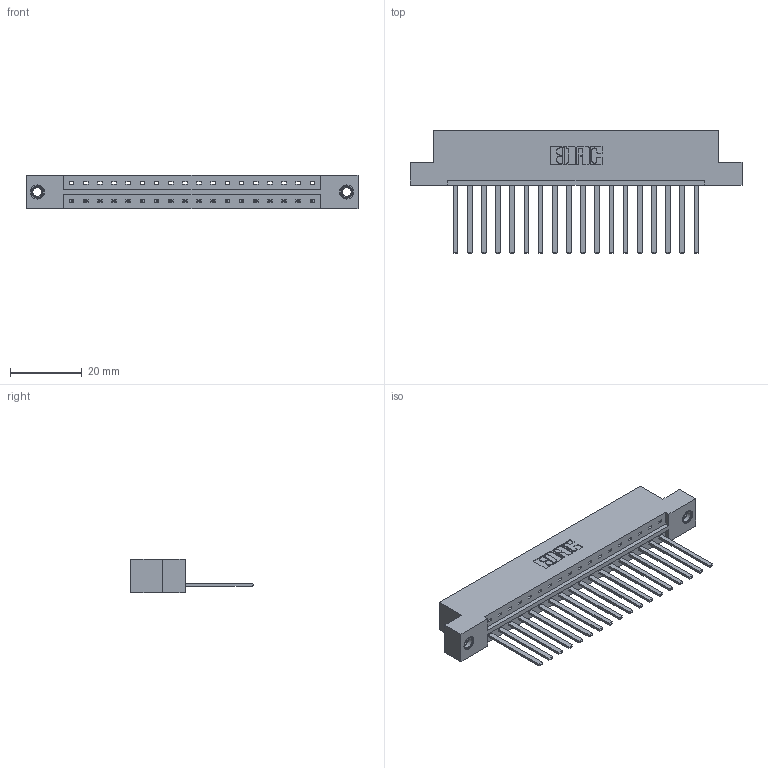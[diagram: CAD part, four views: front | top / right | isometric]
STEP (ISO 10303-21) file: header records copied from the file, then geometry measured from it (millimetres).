
FILE_DESCRIPTION (( 'STEP AP203' ), '1' );
FILE_NAME ('833-018-544-107.STEP', '2020-05-31T22:41:54', ( '' ), ( '' ), 'SwSTEP 2.0', 'SolidWorks 2020', '' );
FILE_SCHEMA (( 'CONFIG_CONTROL_DESIGN' ));
Length unit declared in the file: inch
Products named in the file (4): 833-018-544-107; 345-250-001_345-250-005-103; 833 Part_Flush - .156 Dia - TI; 345-292-001_345-293-144
Assembly tree (21 placements, depth 2):
  833-018-544-107
    833 Part_Flush - .156 Dia - TI
    345-292-001_345-293-144  x18
    345-250-001_345-250-005-103  x2
Bounding box: 92.86 x 34.3 x 9.4 mm (x, y, z)
Volume: 9333.1 mm3; surface area: 10656.6 mm2
Topology: 21 solids, 21 shells, 1110 faces, 3291 edges, 2162 vertices
Faces by surface type: plane 786, cylinder 308, cone 12, torus 4
Entity records: 15110 total; most frequent: CARTESIAN_POINT 2591, ORIENTED_EDGE 2538, DIRECTION 2263, EDGE_CURVE 1269, LINE 1125, VECTOR 1125, VERTEX_POINT 840, AXIS2_PLACEMENT_3D 569
